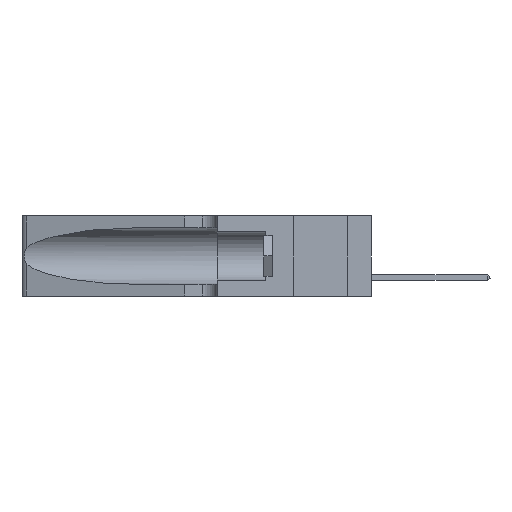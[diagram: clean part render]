
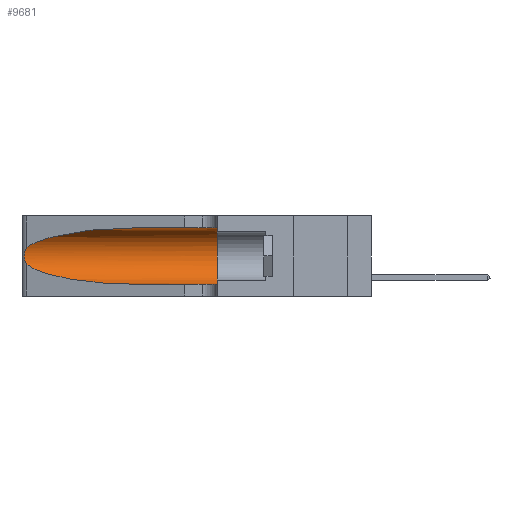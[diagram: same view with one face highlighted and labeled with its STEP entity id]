
A CAD part, left-side view. The second image highlights one B-rep face of the part: STEP entity #9681.
In plain terms, the highlighted cylindrical face has radius 3.308 mm (diameter 6.617 mm), a partial arc.
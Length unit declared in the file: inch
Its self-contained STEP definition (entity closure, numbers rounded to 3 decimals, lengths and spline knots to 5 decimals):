
#404 = ORIENTED_EDGE ( 'NONE', *, *, #25008, .F. ) ;
#762 = VERTEX_POINT ( 'NONE', #45819 ) ;
#1394 = CARTESIAN_POINT ( 'NONE',  ( 0.25487, 1.22718, 0.14631 ) ) ;
#2240 = VERTEX_POINT ( 'NONE', #1394 ) ;
#3340 = AXIS2_PLACEMENT_3D ( 'NONE', #9348, #47224, #18084 ) ;
#3561 = VERTEX_POINT ( 'NONE', #3981 ) ;
#3877 = EDGE_CURVE ( 'NONE', #10612, #2240, #22498, .T. ) ;
#3981 = CARTESIAN_POINT ( 'NONE',  ( 0.1305, 0.35, 0.31525 ) ) ;
#4147 = CARTESIAN_POINT ( 'NONE',  ( 0.18966, 0.96281, 0.05475 ) ) ;
#4300 = DIRECTION ( 'NONE',  ( 0., -1., 0. ) ) ;
#5309 = CARTESIAN_POINT ( 'NONE',  ( 0.1305, 0.35, 0.185 ) ) ;
#7267 = VECTOR ( 'NONE', #8018, 39.37008 ) ;
#8018 = DIRECTION ( 'NONE',  ( 0., -1., 0. ) ) ;
#8476 = CARTESIAN_POINT ( 'NONE',  ( 0.1305, 1.61858, 0.31525 ) ) ;
#8864 = CARTESIAN_POINT ( 'NONE',  ( 0.25487, 1.22718, 0.14631 ) ) ;
#9348 = CARTESIAN_POINT ( 'NONE',  ( 0.1305, 1.61858, 0.185 ) ) ;
#9435 = EDGE_CURVE ( 'NONE', #2240, #35660, #21005, .T. ) ;
#9681 = ADVANCED_FACE ( 'NONE', ( #15907 ), #14207, .F. ) ;
#10612 = VERTEX_POINT ( 'NONE', #28073 ) ;
#12020 = CARTESIAN_POINT ( 'NONE',  ( 0.25856, 1.23593, 0.16098 ) ) ;
#12423 = CARTESIAN_POINT ( 'NONE',  ( 0.25487, 1.22718, 0.22369 ) ) ;
#14207 = CYLINDRICAL_SURFACE ( 'NONE', #3340, 0.13025 ) ;
#14967 = LINE ( 'NONE', #33809, #32000 ) ;
#15907 = FACE_OUTER_BOUND ( 'NONE', #44451, .T. ) ;
#16302 = CARTESIAN_POINT ( 'NONE',  ( 0.25555, 1.22993, 0.14849 ) ) ;
#17781 = ORIENTED_EDGE ( 'NONE', *, *, #25094, .F. ) ;
#18084 = DIRECTION ( 'NONE',  ( 0., 0., -1. ) ) ;
#18502 = CARTESIAN_POINT ( 'NONE',  ( 0.2373, 1.15595, 0.08982 ) ) ;
#20478 = DIRECTION ( 'NONE',  ( 0., 0., 1. ) ) ;
#21005 =( BOUNDED_CURVE ( )  B_SPLINE_CURVE ( 3, ( #37296, #18502, #4147, #44881 ),
 .UNSPECIFIED., .F., .F. ) 
 B_SPLINE_CURVE_WITH_KNOTS ( ( 4, 4 ),
 ( 3.44316, 4.71239 ),
 .UNSPECIFIED. ) 
 CURVE ( )  GEOMETRIC_REPRESENTATION_ITEM ( )  RATIONAL_B_SPLINE_CURVE ( ( 1., 0.87, 0.87, 1. ) ) 
 REPRESENTATION_ITEM ( '' )  );
#21252 = CARTESIAN_POINT ( 'NONE',  ( 0.1305, 0.72297, 0.05475 ) ) ;
#21801 = CARTESIAN_POINT ( 'NONE',  ( 0.25487, 1.22718, 0.22369 ) ) ;
#22278 = CARTESIAN_POINT ( 'NONE',  ( 0.26018, 1.23835, 0.19895 ) ) ;
#22403 = CARTESIAN_POINT ( 'NONE',  ( 0.1305, 0.72297, 0.31525 ) ) ;
#22498 = B_SPLINE_CURVE_WITH_KNOTS ( 'NONE', 3,
 ( #21801, #40773, #44855, #30035, #22604, #22278, #27138, #45472, #26670, #12020, #45796, #23227, #16302, #8864 ),
 .UNSPECIFIED., .F., .F.,
 ( 4, 2, 2, 2, 2, 2, 4 ),
 ( 0., 0.00027, 0.00053, 0.00107, 0.0016, 0.00187, 0.00214 ),
 .UNSPECIFIED. ) ;
#22604 = CARTESIAN_POINT ( 'NONE',  ( 0.25854, 1.2359, 0.20912 ) ) ;
#22628 = ORIENTED_EDGE ( 'NONE', *, *, #9435, .T. ) ;
#23163 = CIRCLE ( 'NONE', #35264, 0.13025 ) ;
#23227 = CARTESIAN_POINT ( 'NONE',  ( 0.25639, 1.23186, 0.15144 ) ) ;
#23823 = ORIENTED_EDGE ( 'NONE', *, *, #43647, .T. ) ;
#24093 = CARTESIAN_POINT ( 'NONE',  ( 0.18966, 0.96281, 0.31525 ) ) ;
#25008 = EDGE_CURVE ( 'NONE', #3561, #762, #23163, .T. ) ;
#25094 = EDGE_CURVE ( 'NONE', #27561, #3561, #30236, .T. ) ;
#26670 = CARTESIAN_POINT ( 'NONE',  ( 0.26017, 1.23833, 0.17102 ) ) ;
#27138 = CARTESIAN_POINT ( 'NONE',  ( 0.26075, 1.23896, 0.19203 ) ) ;
#27291 =( BOUNDED_CURVE ( )  B_SPLINE_CURVE ( 3, ( #46671, #24093, #31364, #12423 ),
 .UNSPECIFIED., .F., .T. ) 
 B_SPLINE_CURVE_WITH_KNOTS ( ( 4, 4 ),
 ( 1.5708, 2.84003 ),
 .UNSPECIFIED. ) 
 CURVE ( )  GEOMETRIC_REPRESENTATION_ITEM ( )  RATIONAL_B_SPLINE_CURVE ( ( 1., 0.87, 0.87, 1. ) ) 
 REPRESENTATION_ITEM ( '' )  );
#27561 = VERTEX_POINT ( 'NONE', #22403 ) ;
#28073 = CARTESIAN_POINT ( 'NONE',  ( 0.25487, 1.22718, 0.22369 ) ) ;
#30035 = CARTESIAN_POINT ( 'NONE',  ( 0.25787, 1.23484, 0.2124 ) ) ;
#30236 = LINE ( 'NONE', #8476, #7267 ) ;
#31364 = CARTESIAN_POINT ( 'NONE',  ( 0.2373, 1.15595, 0.28018 ) ) ;
#32000 = VECTOR ( 'NONE', #4300, 39.37008 ) ;
#33809 = CARTESIAN_POINT ( 'NONE',  ( 0.1305, 1.61858, 0.05475 ) ) ;
#34523 = EDGE_CURVE ( 'NONE', #27561, #10612, #27291, .T. ) ;
#35264 = AXIS2_PLACEMENT_3D ( 'NONE', #5309, #43016, #20478 ) ;
#35660 = VERTEX_POINT ( 'NONE', #21252 ) ;
#37296 = CARTESIAN_POINT ( 'NONE',  ( 0.25487, 1.22718, 0.14631 ) ) ;
#37318 = ORIENTED_EDGE ( 'NONE', *, *, #3877, .T. ) ;
#40773 = CARTESIAN_POINT ( 'NONE',  ( 0.25555, 1.22994, 0.2215 ) ) ;
#43016 = DIRECTION ( 'NONE',  ( 0., 1., 0. ) ) ;
#43647 = EDGE_CURVE ( 'NONE', #35660, #762, #14967, .T. ) ;
#44451 = EDGE_LOOP ( 'NONE', ( #44821, #37318, #22628, #23823, #404, #17781 ) ) ;
#44821 = ORIENTED_EDGE ( 'NONE', *, *, #34523, .T. ) ;
#44855 = CARTESIAN_POINT ( 'NONE',  ( 0.25639, 1.23184, 0.21858 ) ) ;
#44881 = CARTESIAN_POINT ( 'NONE',  ( 0.1305, 0.72297, 0.05475 ) ) ;
#45472 = CARTESIAN_POINT ( 'NONE',  ( 0.26075, 1.23896, 0.178 ) ) ;
#45796 = CARTESIAN_POINT ( 'NONE',  ( 0.25789, 1.23486, 0.15765 ) ) ;
#45819 = CARTESIAN_POINT ( 'NONE',  ( 0.1305, 0.35, 0.05475 ) ) ;
#46671 = CARTESIAN_POINT ( 'NONE',  ( 0.1305, 0.72297, 0.31525 ) ) ;
#47224 = DIRECTION ( 'NONE',  ( 0., -1., 0. ) ) ;
